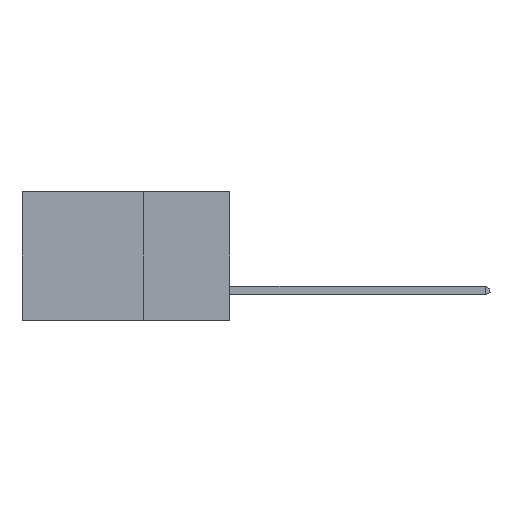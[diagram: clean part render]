
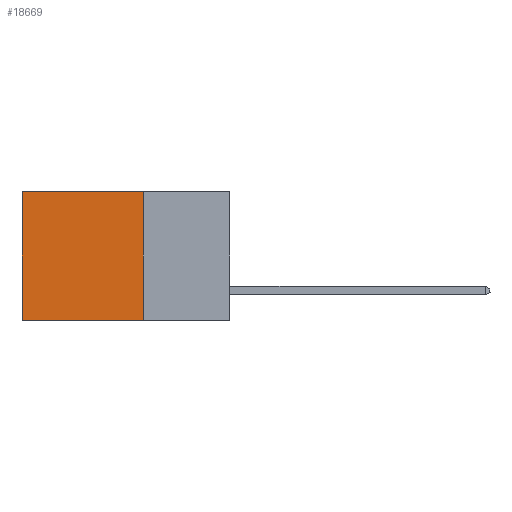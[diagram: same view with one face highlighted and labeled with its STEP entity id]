
A CAD part, left-side view. The second image highlights one B-rep face of the part: STEP entity #18669.
In plain terms, the highlighted planar face has unit normal (-1, 0, 0).
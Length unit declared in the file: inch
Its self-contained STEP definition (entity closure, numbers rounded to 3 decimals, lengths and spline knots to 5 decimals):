
#891 = CARTESIAN_POINT ( 'NONE',  ( 0.298, 0.25, 0. ) ) ;
#1149 = DIRECTION ( 'NONE',  ( 0., 0., -1. ) ) ;
#1252 = VERTEX_POINT ( 'NONE', #10377 ) ;
#1609 = VERTEX_POINT ( 'NONE', #15541 ) ;
#1773 = CARTESIAN_POINT ( 'NONE',  ( 0.298, 0.25, 0. ) ) ;
#2343 = EDGE_CURVE ( 'NONE', #3941, #1609, #2389, .T. ) ;
#2389 = LINE ( 'NONE', #13964, #9627 ) ;
#2669 = EDGE_CURVE ( 'NONE', #1252, #1609, #5339, .T. ) ;
#3030 = ORIENTED_EDGE ( 'NONE', *, *, #11857, .F. ) ;
#3588 = DIRECTION ( 'NONE',  ( 1., 0., 0. ) ) ;
#3620 = FACE_OUTER_BOUND ( 'NONE', #12228, .T. ) ;
#3651 = LINE ( 'NONE', #6238, #8838 ) ;
#3941 = VERTEX_POINT ( 'NONE', #9630 ) ;
#4557 = DIRECTION ( 'NONE',  ( 0., 0., -1. ) ) ;
#5339 = LINE ( 'NONE', #9846, #17061 ) ;
#6238 = CARTESIAN_POINT ( 'NONE',  ( 0.298, 0.25, 0. ) ) ;
#6600 = DIRECTION ( 'NONE',  ( 0., 0., -1. ) ) ;
#8223 = DIRECTION ( 'NONE',  ( 0., 1., 0. ) ) ;
#8331 = ORIENTED_EDGE ( 'NONE', *, *, #2669, .T. ) ;
#8838 = VECTOR ( 'NONE', #4557, 39.37008 ) ;
#9427 = CARTESIAN_POINT ( 'NONE',  ( 0.298, 0.25, 0. ) ) ;
#9627 = VECTOR ( 'NONE', #8223, 39.37008 ) ;
#9630 = CARTESIAN_POINT ( 'NONE',  ( 0.298, 0.25, -0.37 ) ) ;
#9846 = CARTESIAN_POINT ( 'NONE',  ( 0.298, 0.6, 0. ) ) ;
#10377 = CARTESIAN_POINT ( 'NONE',  ( 0.298, 0.6, 0. ) ) ;
#10917 = PLANE ( 'NONE',  #18720 ) ;
#10925 = LINE ( 'NONE', #1773, #14304 ) ;
#11857 = EDGE_CURVE ( 'NONE', #13471, #3941, #3651, .T. ) ;
#12228 = EDGE_LOOP ( 'NONE', ( #8331, #15770, #3030, #17636 ) ) ;
#13469 = DIRECTION ( 'NONE',  ( 0., 1., 0. ) ) ;
#13471 = VERTEX_POINT ( 'NONE', #9427 ) ;
#13964 = CARTESIAN_POINT ( 'NONE',  ( 0.298, 0.25, -0.37 ) ) ;
#14304 = VECTOR ( 'NONE', #13469, 39.37008 ) ;
#15541 = CARTESIAN_POINT ( 'NONE',  ( 0.298, 0.6, -0.37 ) ) ;
#15770 = ORIENTED_EDGE ( 'NONE', *, *, #2343, .F. ) ;
#16943 = EDGE_CURVE ( 'NONE', #13471, #1252, #10925, .T. ) ;
#17061 = VECTOR ( 'NONE', #1149, 39.37008 ) ;
#17636 = ORIENTED_EDGE ( 'NONE', *, *, #16943, .T. ) ;
#18669 = ADVANCED_FACE ( 'NONE', ( #3620 ), #10917, .F. ) ;
#18720 = AXIS2_PLACEMENT_3D ( 'NONE', #891, #3588, #6600 ) ;
